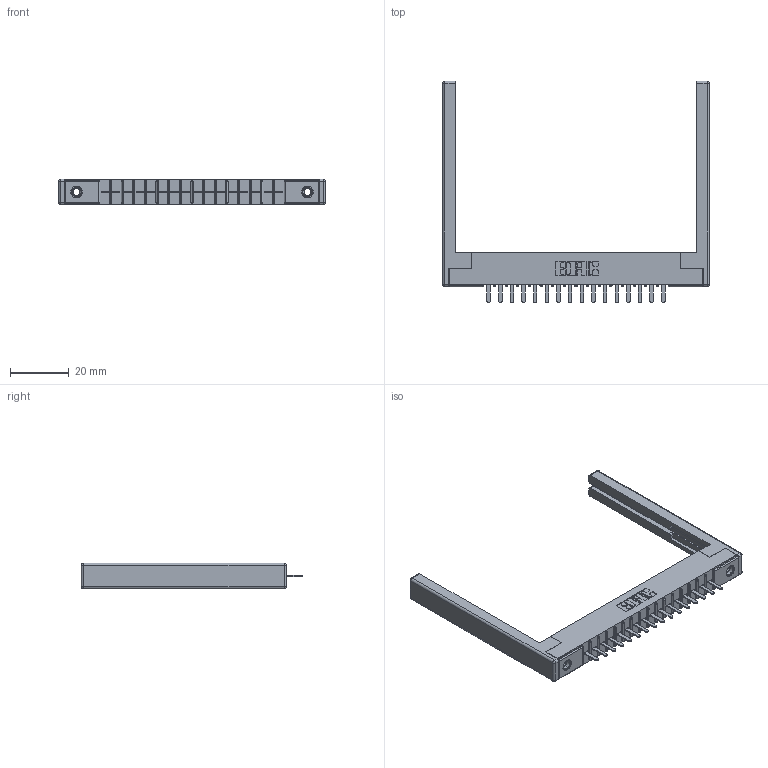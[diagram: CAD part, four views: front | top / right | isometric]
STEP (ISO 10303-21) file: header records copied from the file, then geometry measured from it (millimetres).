
FILE_DESCRIPTION (( 'STEP AP203' ), '1' );
FILE_NAME ('306-016-520-168.STEP', '2019-09-11T20:06:51', ( '' ), ( '' ), 'SwSTEP 2.0', 'SolidWorks 2016', '' );
FILE_SCHEMA (( 'CONFIG_CONTROL_DESIGN' ));
Length unit declared in the file: inch
Products named in the file (5): 345-250-001_345-250-001-102; 307-220-068; 306-016-520-168; 306 Part_.156 Dia; 306-290-001_120
Assembly tree (21 placements, depth 2):
  306-016-520-168
    306 Part_.156 Dia
    306-290-001_120  x16
    345-250-001_345-250-001-102  x2
    307-220-068  x2
Bounding box: 90.83 x 75.41 x 8.71 mm (x, y, z)
Volume: 10732.2 mm3; surface area: 13077.7 mm2
Topology: 21 solids, 21 shells, 1390 faces, 3858 edges, 2464 vertices
Faces by surface type: plane 908, cylinder 394, sphere 72, cone 12, torus 4
Entity records: 21004 total; most frequent: CARTESIAN_POINT 3488, DIRECTION 3455, ORIENTED_EDGE 3446, EDGE_CURVE 1723, LINE 1329, VECTOR 1329, VERTEX_POINT 1096, AXIS2_PLACEMENT_3D 1063
